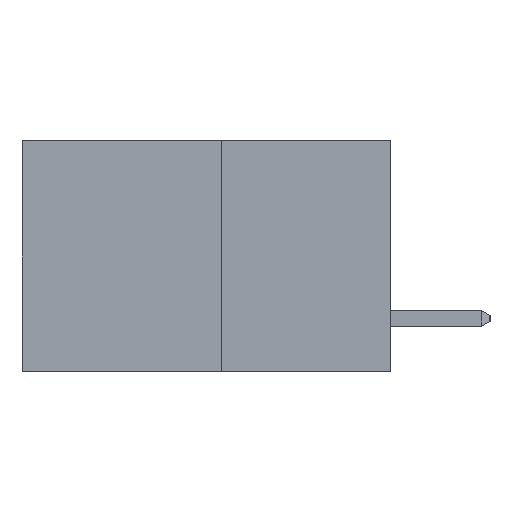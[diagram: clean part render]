
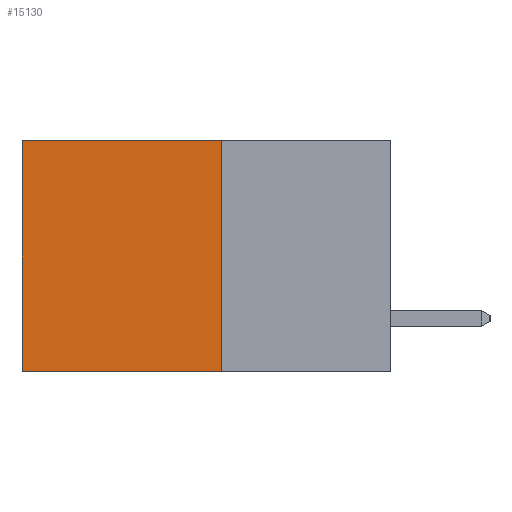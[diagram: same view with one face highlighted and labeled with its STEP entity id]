
A CAD part, left-side view. The second image highlights one B-rep face of the part: STEP entity #15130.
In plain terms, the highlighted planar face has unit normal (-1, 0, 0).
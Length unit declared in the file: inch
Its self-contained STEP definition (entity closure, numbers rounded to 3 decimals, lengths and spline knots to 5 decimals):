
#1896 = VERTEX_POINT ( 'NONE', #14995 ) ;
#4333 = EDGE_CURVE ( 'NONE', #4750, #1896, #5450, .T. ) ;
#4750 = VERTEX_POINT ( 'NONE', #19957 ) ;
#4813 = DIRECTION ( 'NONE',  ( 0., 0., -1. ) ) ;
#4880 = CARTESIAN_POINT ( 'NONE',  ( 0.277, 0.59, -0.37 ) ) ;
#5450 = LINE ( 'NONE', #15759, #13071 ) ;
#6179 = ORIENTED_EDGE ( 'NONE', *, *, #16354, .F. ) ;
#6519 = FACE_OUTER_BOUND ( 'NONE', #19979, .T. ) ;
#8279 = AXIS2_PLACEMENT_3D ( 'NONE', #16436, #19623, #10001 ) ;
#10001 = DIRECTION ( 'NONE',  ( 0., 0., -1. ) ) ;
#10123 = ORIENTED_EDGE ( 'NONE', *, *, #15037, .T. ) ;
#10210 = CARTESIAN_POINT ( 'NONE',  ( 0.277, 0.27, -0.37 ) ) ;
#11842 = VECTOR ( 'NONE', #14032, 39.37008 ) ;
#12103 = LINE ( 'NONE', #10210, #15923 ) ;
#12203 = VERTEX_POINT ( 'NONE', #13646 ) ;
#12381 = LINE ( 'NONE', #4880, #20899 ) ;
#13071 = VECTOR ( 'NONE', #15823, 39.37008 ) ;
#13646 = CARTESIAN_POINT ( 'NONE',  ( 0.277, 0.59, 0. ) ) ;
#14032 = DIRECTION ( 'NONE',  ( 0., 1., 0. ) ) ;
#14198 = ORIENTED_EDGE ( 'NONE', *, *, #4333, .F. ) ;
#14823 = PLANE ( 'NONE',  #8279 ) ;
#14995 = CARTESIAN_POINT ( 'NONE',  ( 0.277, 0.59, -0.37 ) ) ;
#15037 = EDGE_CURVE ( 'NONE', #12203, #1896, #12381, .T. ) ;
#15130 = ADVANCED_FACE ( 'NONE', ( #6519 ), #14823, .F. ) ;
#15759 = CARTESIAN_POINT ( 'NONE',  ( 0.277, 0.27, -0.37 ) ) ;
#15823 = DIRECTION ( 'NONE',  ( 0., 1., 0. ) ) ;
#15904 = EDGE_CURVE ( 'NONE', #20819, #12203, #16158, .T. ) ;
#15923 = VECTOR ( 'NONE', #19809, 39.37008 ) ;
#16158 = LINE ( 'NONE', #20375, #11842 ) ;
#16354 = EDGE_CURVE ( 'NONE', #20819, #4750, #12103, .T. ) ;
#16436 = CARTESIAN_POINT ( 'NONE',  ( 0.277, 0.27, -0.37 ) ) ;
#17283 = ORIENTED_EDGE ( 'NONE', *, *, #15904, .T. ) ;
#18371 = CARTESIAN_POINT ( 'NONE',  ( 0.277, 0.27, 0. ) ) ;
#19623 = DIRECTION ( 'NONE',  ( 1., 0., 0. ) ) ;
#19809 = DIRECTION ( 'NONE',  ( 0., 0., -1. ) ) ;
#19957 = CARTESIAN_POINT ( 'NONE',  ( 0.277, 0.27, -0.37 ) ) ;
#19979 = EDGE_LOOP ( 'NONE', ( #10123, #14198, #6179, #17283 ) ) ;
#20375 = CARTESIAN_POINT ( 'NONE',  ( 0.277, 0.27, 0. ) ) ;
#20819 = VERTEX_POINT ( 'NONE', #18371 ) ;
#20899 = VECTOR ( 'NONE', #4813, 39.37008 ) ;
